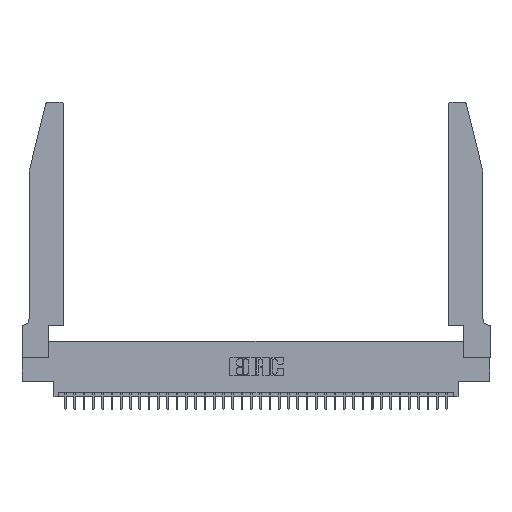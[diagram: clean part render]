
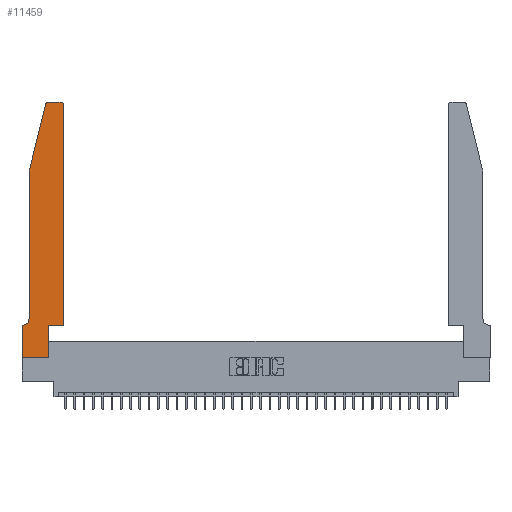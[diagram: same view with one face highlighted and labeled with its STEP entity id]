
A CAD part, top view. The second image highlights one B-rep face of the part: STEP entity #11459.
In plain terms, the highlighted planar face has unit normal (0, 0, 1).
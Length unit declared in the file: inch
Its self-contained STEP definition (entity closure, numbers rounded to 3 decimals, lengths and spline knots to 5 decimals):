
#152 = VERTEX_POINT ( 'NONE', #23375 ) ;
#335 = AXIS2_PLACEMENT_3D ( 'NONE', #3446, #14987, #568 ) ;
#568 = DIRECTION ( 'NONE',  ( -1., 0., 0. ) ) ;
#742 = CARTESIAN_POINT ( 'NONE',  ( 0.0755, 0.42, 0.37 ) ) ;
#1323 = AXIS2_PLACEMENT_3D ( 'NONE', #13871, #7706, #7490 ) ;
#1361 = LINE ( 'NONE', #36478, #30971 ) ;
#1665 = CARTESIAN_POINT ( 'NONE',  ( 0.4505, 0.35, 0.37 ) ) ;
#1707 = DIRECTION ( 'NONE',  ( 1., 0., 0. ) ) ;
#1738 = ORIENTED_EDGE ( 'NONE', *, *, #10910, .T. ) ;
#1868 = CARTESIAN_POINT ( 'NONE',  ( 0.2865, 0.35, 0.37 ) ) ;
#2869 = AXIS2_PLACEMENT_3D ( 'NONE', #37914, #34858, #20694 ) ;
#2998 = VERTEX_POINT ( 'NONE', #34786 ) ;
#3323 = VERTEX_POINT ( 'NONE', #1665 ) ;
#3446 = CARTESIAN_POINT ( 'NONE',  ( 0.0055, 0.42, 0.37 ) ) ;
#3675 = LINE ( 'NONE', #9440, #31890 ) ;
#4022 = VECTOR ( 'NONE', #8579, 39.37008 ) ;
#4606 = DIRECTION ( 'NONE',  ( -1., 0., 0. ) ) ;
#5462 = FACE_OUTER_BOUND ( 'NONE', #34120, .T. ) ;
#5944 = ORIENTED_EDGE ( 'NONE', *, *, #6041, .T. ) ;
#6041 = EDGE_CURVE ( 'NONE', #31803, #26027, #3675, .T. ) ;
#6736 = VERTEX_POINT ( 'NONE', #32021 ) ;
#6886 = VECTOR ( 'NONE', #28527, 39.37008 ) ;
#7042 = ORIENTED_EDGE ( 'NONE', *, *, #26071, .T. ) ;
#7120 = ORIENTED_EDGE ( 'NONE', *, *, #22572, .T. ) ;
#7273 = CARTESIAN_POINT ( 'NONE',  ( 0.4205, 2.75, 0.37 ) ) ;
#7385 = CARTESIAN_POINT ( 'NONE',  ( 0.25487, 2.72718, 0.37 ) ) ;
#7490 = DIRECTION ( 'NONE',  ( 1., 0., 0. ) ) ;
#7706 = DIRECTION ( 'NONE',  ( 0., 0., 1. ) ) ;
#8214 = DIRECTION ( 'NONE',  ( -1., 0., 0. ) ) ;
#8439 = EDGE_CURVE ( 'NONE', #2998, #14391, #36680, .T. ) ;
#8579 = DIRECTION ( 'NONE',  ( 1., 0., 0. ) ) ;
#9405 = ORIENTED_EDGE ( 'NONE', *, *, #19615, .T. ) ;
#9440 = CARTESIAN_POINT ( 'NONE',  ( 0.0755, 2., 0.37 ) ) ;
#9480 = CIRCLE ( 'NONE', #30955, 0.03 ) ;
#9914 = ORIENTED_EDGE ( 'NONE', *, *, #12786, .T. ) ;
#10693 = CARTESIAN_POINT ( 'NONE',  ( 0.4505, 0.35, 0.37 ) ) ;
#10910 = EDGE_CURVE ( 'NONE', #33275, #33887, #16188, .T. ) ;
#11322 = CARTESIAN_POINT ( 'NONE',  ( 0.2865, 0.35, 0.37 ) ) ;
#11459 = ADVANCED_FACE ( 'NONE', ( #5462 ), #29290, .T. ) ;
#11642 = LINE ( 'NONE', #17469, #4022 ) ;
#11922 = CARTESIAN_POINT ( 'NONE',  ( 0.284, 2.72, 0.37 ) ) ;
#12050 = EDGE_CURVE ( 'NONE', #33887, #23950, #9480, .T. ) ;
#12786 = EDGE_CURVE ( 'NONE', #152, #29265, #25344, .T. ) ;
#12853 = VERTEX_POINT ( 'NONE', #14714 ) ;
#13320 = CARTESIAN_POINT ( 'NONE',  ( 0.4505, 0.35, 0.37 ) ) ;
#13778 = DIRECTION ( 'NONE',  ( 0., 1., 0. ) ) ;
#13871 = CARTESIAN_POINT ( 'NONE',  ( 0.4205, 2.72, 0.37 ) ) ;
#13877 = ORIENTED_EDGE ( 'NONE', *, *, #12050, .T. ) ;
#14391 = VERTEX_POINT ( 'NONE', #25227 ) ;
#14434 = CIRCLE ( 'NONE', #335, 0.07 ) ;
#14714 = CARTESIAN_POINT ( 'NONE',  ( 0.4505, 2.72, 0.37 ) ) ;
#14987 = DIRECTION ( 'NONE',  ( 0., 0., -1. ) ) ;
#15512 = LINE ( 'NONE', #24386, #22217 ) ;
#15619 = EDGE_CURVE ( 'NONE', #12853, #33275, #20982, .T. ) ;
#16060 = ORIENTED_EDGE ( 'NONE', *, *, #8439, .T. ) ;
#16188 = LINE ( 'NONE', #36670, #31322 ) ;
#16583 = EDGE_CURVE ( 'NONE', #3323, #12853, #25286, .T. ) ;
#17469 = CARTESIAN_POINT ( 'NONE',  ( 0., 0., 0.37 ) ) ;
#18406 = DIRECTION ( 'NONE',  ( -0.239, -0.971, 0. ) ) ;
#19615 = EDGE_CURVE ( 'NONE', #26027, #2998, #14434, .T. ) ;
#20009 = ORIENTED_EDGE ( 'NONE', *, *, #15619, .T. ) ;
#20694 = DIRECTION ( 'NONE',  ( 1., 0., 0. ) ) ;
#20982 = CIRCLE ( 'NONE', #1323, 0.03 ) ;
#22217 = VECTOR ( 'NONE', #18406, 39.37008 ) ;
#22275 = LINE ( 'NONE', #10693, #26969 ) ;
#22572 = EDGE_CURVE ( 'NONE', #6736, #152, #11642, .T. ) ;
#23375 = CARTESIAN_POINT ( 'NONE',  ( 0.2865, 0., 0.37 ) ) ;
#23950 = VERTEX_POINT ( 'NONE', #7385 ) ;
#24386 = CARTESIAN_POINT ( 'NONE',  ( 0.0755, 2., 0.37 ) ) ;
#25227 = CARTESIAN_POINT ( 'NONE',  ( 0., 0.35, 0.37 ) ) ;
#25286 = LINE ( 'NONE', #13320, #6886 ) ;
#25344 = LINE ( 'NONE', #1868, #29501 ) ;
#26027 = VERTEX_POINT ( 'NONE', #742 ) ;
#26071 = EDGE_CURVE ( 'NONE', #29265, #3323, #22275, .T. ) ;
#26795 = DIRECTION ( 'NONE',  ( 0., 0., 1. ) ) ;
#26969 = VECTOR ( 'NONE', #1707, 39.37008 ) ;
#27083 = ORIENTED_EDGE ( 'NONE', *, *, #16583, .T. ) ;
#27466 = EDGE_CURVE ( 'NONE', #23950, #31803, #15512, .T. ) ;
#28527 = DIRECTION ( 'NONE',  ( 0., 1., 0. ) ) ;
#29265 = VERTEX_POINT ( 'NONE', #11322 ) ;
#29290 = PLANE ( 'NONE',  #2869 ) ;
#29501 = VECTOR ( 'NONE', #13778, 39.37008 ) ;
#29980 = DIRECTION ( 'NONE',  ( 1., 0., 0. ) ) ;
#30127 = ORIENTED_EDGE ( 'NONE', *, *, #33379, .T. ) ;
#30931 = CARTESIAN_POINT ( 'NONE',  ( 0.0755, 0.35, 0.37 ) ) ;
#30955 = AXIS2_PLACEMENT_3D ( 'NONE', #11922, #26795, #29980 ) ;
#30971 = VECTOR ( 'NONE', #37430, 39.37008 ) ;
#31322 = VECTOR ( 'NONE', #8214, 39.37008 ) ;
#31563 = ORIENTED_EDGE ( 'NONE', *, *, #27466, .T. ) ;
#31803 = VERTEX_POINT ( 'NONE', #33060 ) ;
#31890 = VECTOR ( 'NONE', #35571, 39.37008 ) ;
#32021 = CARTESIAN_POINT ( 'NONE',  ( 0., 0., 0.37 ) ) ;
#33060 = CARTESIAN_POINT ( 'NONE',  ( 0.0755, 2., 0.37 ) ) ;
#33275 = VERTEX_POINT ( 'NONE', #7273 ) ;
#33379 = EDGE_CURVE ( 'NONE', #14391, #6736, #1361, .T. ) ;
#33887 = VERTEX_POINT ( 'NONE', #34534 ) ;
#34120 = EDGE_LOOP ( 'NONE', ( #1738, #13877, #31563, #5944, #9405, #16060, #30127, #7120, #9914, #7042, #27083, #20009 ) ) ;
#34534 = CARTESIAN_POINT ( 'NONE',  ( 0.284, 2.75, 0.37 ) ) ;
#34786 = CARTESIAN_POINT ( 'NONE',  ( 0.0055, 0.35, 0.37 ) ) ;
#34858 = DIRECTION ( 'NONE',  ( 0., 0., 1. ) ) ;
#35571 = DIRECTION ( 'NONE',  ( 0., -1., 0. ) ) ;
#36478 = CARTESIAN_POINT ( 'NONE',  ( 0., 0., 0.37 ) ) ;
#36670 = CARTESIAN_POINT ( 'NONE',  ( 0.2605, 2.75, 0.37 ) ) ;
#36680 = LINE ( 'NONE', #30931, #37328 ) ;
#37328 = VECTOR ( 'NONE', #4606, 39.37008 ) ;
#37430 = DIRECTION ( 'NONE',  ( 0., -1., 0. ) ) ;
#37914 = CARTESIAN_POINT ( 'NONE',  ( 0., 0.35, 0.37 ) ) ;
